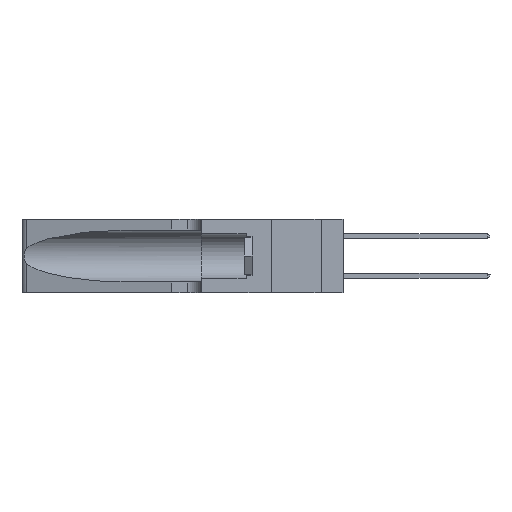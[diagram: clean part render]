
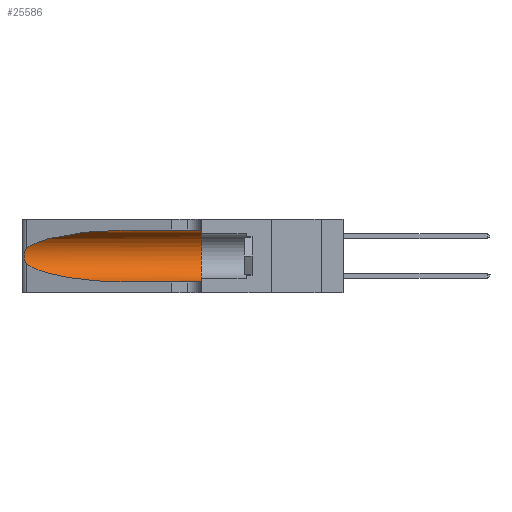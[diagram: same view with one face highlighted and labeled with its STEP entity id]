
A CAD part, left-side view. The second image highlights one B-rep face of the part: STEP entity #25586.
In plain terms, the highlighted cylindrical face has radius 3.308 mm (diameter 6.617 mm), a partial arc.
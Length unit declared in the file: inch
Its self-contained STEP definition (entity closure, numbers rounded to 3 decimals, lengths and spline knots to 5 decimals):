
#310 = VECTOR ( 'NONE', #25423, 39.37008 ) ;
#923 = CARTESIAN_POINT ( 'NONE',  ( 0.26017, 1.23833, 0.17102 ) ) ;
#968 = CARTESIAN_POINT ( 'NONE',  ( 0.1305, 0.35, 0.185 ) ) ;
#1019 = EDGE_LOOP ( 'NONE', ( #8931, #5549, #7674, #11096, #27289, #16120 ) ) ;
#1172 = DIRECTION ( 'NONE',  ( 0., -1., 0. ) ) ;
#2468 = CARTESIAN_POINT ( 'NONE',  ( 0.25487, 1.22718, 0.14631 ) ) ;
#2536 = EDGE_CURVE ( 'NONE', #11702, #10621, #13958, .T. ) ;
#2562 = VERTEX_POINT ( 'NONE', #3318 ) ;
#2579 = CARTESIAN_POINT ( 'NONE',  ( 0.2373, 1.15595, 0.08982 ) ) ;
#3179 = CARTESIAN_POINT ( 'NONE',  ( 0.25789, 1.23486, 0.15765 ) ) ;
#3221 = DIRECTION ( 'NONE',  ( 0., 0., 1. ) ) ;
#3273 = CARTESIAN_POINT ( 'NONE',  ( 0.1305, 0.35, 0.31525 ) ) ;
#3318 = CARTESIAN_POINT ( 'NONE',  ( 0.1305, 0.72297, 0.31525 ) ) ;
#3958 = EDGE_CURVE ( 'NONE', #2562, #11702, #16535, .T. ) ;
#4134 = CARTESIAN_POINT ( 'NONE',  ( 0.1305, 0.35, 0.05475 ) ) ;
#4789 = CARTESIAN_POINT ( 'NONE',  ( 0.18966, 0.96281, 0.05475 ) ) ;
#5101 = AXIS2_PLACEMENT_3D ( 'NONE', #27200, #1172, #12214 ) ;
#5384 = CARTESIAN_POINT ( 'NONE',  ( 0.25555, 1.22993, 0.14849 ) ) ;
#5549 = ORIENTED_EDGE ( 'NONE', *, *, #13491, .T. ) ;
#5856 = CARTESIAN_POINT ( 'NONE',  ( 0.1305, 1.61858, 0.31525 ) ) ;
#6429 = DIRECTION ( 'NONE',  ( 0., -1., 0. ) ) ;
#6565 = CYLINDRICAL_SURFACE ( 'NONE', #5101, 0.13025 ) ;
#6661 = CARTESIAN_POINT ( 'NONE',  ( 0.18966, 0.96281, 0.31525 ) ) ;
#7487 = CARTESIAN_POINT ( 'NONE',  ( 0.25555, 1.22994, 0.2215 ) ) ;
#7674 = ORIENTED_EDGE ( 'NONE', *, *, #15871, .T. ) ;
#8744 = EDGE_CURVE ( 'NONE', #21541, #10621, #16294, .T. ) ;
#8871 = VERTEX_POINT ( 'NONE', #2468 ) ;
#8931 = ORIENTED_EDGE ( 'NONE', *, *, #21195, .T. ) ;
#8968 = VERTEX_POINT ( 'NONE', #9440 ) ;
#9440 = CARTESIAN_POINT ( 'NONE',  ( 0.25487, 1.22718, 0.22369 ) ) ;
#9755 = CARTESIAN_POINT ( 'NONE',  ( 0.25787, 1.23484, 0.2124 ) ) ;
#10621 = VERTEX_POINT ( 'NONE', #4134 ) ;
#11096 = ORIENTED_EDGE ( 'NONE', *, *, #8744, .T. ) ;
#11128 = CARTESIAN_POINT ( 'NONE',  ( 0.2373, 1.15595, 0.28018 ) ) ;
#11702 = VERTEX_POINT ( 'NONE', #3273 ) ;
#11768 = FACE_OUTER_BOUND ( 'NONE', #1019, .T. ) ;
#11961 = CARTESIAN_POINT ( 'NONE',  ( 0.26018, 1.23835, 0.19895 ) ) ;
#12214 = DIRECTION ( 'NONE',  ( 0., 0., -1. ) ) ;
#12338 = AXIS2_PLACEMENT_3D ( 'NONE', #968, #16390, #3221 ) ;
#13117 =( BOUNDED_CURVE ( )  B_SPLINE_CURVE ( 3, ( #15753, #2579, #4789, #20069 ),
 .UNSPECIFIED., .F., .F. ) 
 B_SPLINE_CURVE_WITH_KNOTS ( ( 4, 4 ),
 ( 3.44316, 4.71239 ),
 .UNSPECIFIED. ) 
 CURVE ( )  GEOMETRIC_REPRESENTATION_ITEM ( )  RATIONAL_B_SPLINE_CURVE ( ( 1., 0.87, 0.87, 1. ) ) 
 REPRESENTATION_ITEM ( '' )  );
#13491 = EDGE_CURVE ( 'NONE', #8968, #8871, #18160, .T. ) ;
#13958 = CIRCLE ( 'NONE', #12338, 0.13025 ) ;
#14149 = CARTESIAN_POINT ( 'NONE',  ( 0.26075, 1.23896, 0.178 ) ) ;
#15753 = CARTESIAN_POINT ( 'NONE',  ( 0.25487, 1.22718, 0.14631 ) ) ;
#15871 = EDGE_CURVE ( 'NONE', #8871, #21541, #13117, .T. ) ;
#16120 = ORIENTED_EDGE ( 'NONE', *, *, #3958, .F. ) ;
#16294 = LINE ( 'NONE', #21673, #16986 ) ;
#16348 = CARTESIAN_POINT ( 'NONE',  ( 0.25856, 1.23593, 0.16098 ) ) ;
#16390 = DIRECTION ( 'NONE',  ( 0., 1., 0. ) ) ;
#16535 = LINE ( 'NONE', #5856, #310 ) ;
#16986 = VECTOR ( 'NONE', #6429, 39.37008 ) ;
#18160 = B_SPLINE_CURVE_WITH_KNOTS ( 'NONE', 3,
 ( #20550, #7487, #22704, #9755, #24862, #11961, #26972, #14149, #923, #16348, #3179, #18508, #5384, #20649 ),
 .UNSPECIFIED., .F., .F.,
 ( 4, 2, 2, 2, 2, 2, 4 ),
 ( 0., 0.00027, 0.00053, 0.00107, 0.0016, 0.00187, 0.00214 ),
 .UNSPECIFIED. ) ;
#18508 = CARTESIAN_POINT ( 'NONE',  ( 0.25639, 1.23186, 0.15144 ) ) ;
#18784 = CARTESIAN_POINT ( 'NONE',  ( 0.1305, 0.72297, 0.05475 ) ) ;
#20069 = CARTESIAN_POINT ( 'NONE',  ( 0.1305, 0.72297, 0.05475 ) ) ;
#20550 = CARTESIAN_POINT ( 'NONE',  ( 0.25487, 1.22718, 0.22369 ) ) ;
#20649 = CARTESIAN_POINT ( 'NONE',  ( 0.25487, 1.22718, 0.14631 ) ) ;
#21070 =( BOUNDED_CURVE ( )  B_SPLINE_CURVE ( 3, ( #21901, #6661, #11128, #26177 ),
 .UNSPECIFIED., .F., .T. ) 
 B_SPLINE_CURVE_WITH_KNOTS ( ( 4, 4 ),
 ( 1.5708, 2.84003 ),
 .UNSPECIFIED. ) 
 CURVE ( )  GEOMETRIC_REPRESENTATION_ITEM ( )  RATIONAL_B_SPLINE_CURVE ( ( 1., 0.87, 0.87, 1. ) ) 
 REPRESENTATION_ITEM ( '' )  );
#21195 = EDGE_CURVE ( 'NONE', #2562, #8968, #21070, .T. ) ;
#21541 = VERTEX_POINT ( 'NONE', #18784 ) ;
#21673 = CARTESIAN_POINT ( 'NONE',  ( 0.1305, 1.61858, 0.05475 ) ) ;
#21901 = CARTESIAN_POINT ( 'NONE',  ( 0.1305, 0.72297, 0.31525 ) ) ;
#22704 = CARTESIAN_POINT ( 'NONE',  ( 0.25639, 1.23184, 0.21858 ) ) ;
#24862 = CARTESIAN_POINT ( 'NONE',  ( 0.25854, 1.2359, 0.20912 ) ) ;
#25423 = DIRECTION ( 'NONE',  ( 0., -1., 0. ) ) ;
#25586 = ADVANCED_FACE ( 'NONE', ( #11768 ), #6565, .F. ) ;
#26177 = CARTESIAN_POINT ( 'NONE',  ( 0.25487, 1.22718, 0.22369 ) ) ;
#26972 = CARTESIAN_POINT ( 'NONE',  ( 0.26075, 1.23896, 0.19203 ) ) ;
#27200 = CARTESIAN_POINT ( 'NONE',  ( 0.1305, 1.61858, 0.185 ) ) ;
#27289 = ORIENTED_EDGE ( 'NONE', *, *, #2536, .F. ) ;
